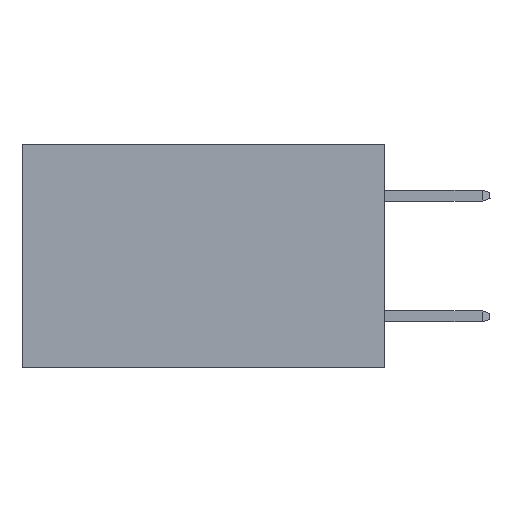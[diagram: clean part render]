
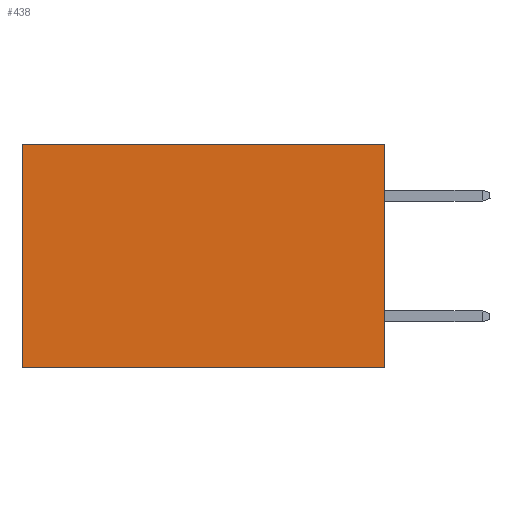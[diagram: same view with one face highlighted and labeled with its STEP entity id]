
A CAD part, left-side view. The second image highlights one B-rep face of the part: STEP entity #438.
In plain terms, the highlighted planar face has unit normal (-1, 0, 0).
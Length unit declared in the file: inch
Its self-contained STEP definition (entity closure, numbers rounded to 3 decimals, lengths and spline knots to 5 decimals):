
#314 = LINE ( 'NONE', #13650, #6365 ) ;
#370 = DIRECTION ( 'NONE',  ( 0., 1., 0. ) ) ;
#438 = ADVANCED_FACE ( 'NONE', ( #1884 ), #11918, .F. ) ;
#947 = CARTESIAN_POINT ( 'NONE',  ( 0.298, 0.6, 0. ) ) ;
#1336 = ORIENTED_EDGE ( 'NONE', *, *, #12572, .F. ) ;
#1884 = FACE_OUTER_BOUND ( 'NONE', #7012, .T. ) ;
#2105 = CARTESIAN_POINT ( 'NONE',  ( 0.298, 0.6, 0. ) ) ;
#2385 = VECTOR ( 'NONE', #9406, 39.37008 ) ;
#2459 = ORIENTED_EDGE ( 'NONE', *, *, #11567, .T. ) ;
#4093 = CARTESIAN_POINT ( 'NONE',  ( 0.298, 0., -0.37 ) ) ;
#4707 = VECTOR ( 'NONE', #14517, 39.37008 ) ;
#4843 = LINE ( 'NONE', #4093, #15502 ) ;
#4847 = DIRECTION ( 'NONE',  ( 0., 0., -1. ) ) ;
#5023 = CARTESIAN_POINT ( 'NONE',  ( 0.298, 0., -0.37 ) ) ;
#6365 = VECTOR ( 'NONE', #12545, 39.37008 ) ;
#6656 = VERTEX_POINT ( 'NONE', #5023 ) ;
#6680 = VERTEX_POINT ( 'NONE', #7475 ) ;
#6783 = LINE ( 'NONE', #9624, #4707 ) ;
#7012 = EDGE_LOOP ( 'NONE', ( #2459, #1336, #11537, #7087 ) ) ;
#7087 = ORIENTED_EDGE ( 'NONE', *, *, #10410, .T. ) ;
#7222 = CARTESIAN_POINT ( 'NONE',  ( 0.298, 0., 0. ) ) ;
#7475 = CARTESIAN_POINT ( 'NONE',  ( 0.298, 0.6, -0.37 ) ) ;
#9406 = DIRECTION ( 'NONE',  ( 0., 0., -1. ) ) ;
#9624 = CARTESIAN_POINT ( 'NONE',  ( 0.298, 0., 0. ) ) ;
#10410 = EDGE_CURVE ( 'NONE', #11607, #10759, #6783, .T. ) ;
#10686 = CARTESIAN_POINT ( 'NONE',  ( 0.298, 0., 0. ) ) ;
#10759 = VERTEX_POINT ( 'NONE', #2105 ) ;
#10783 = DIRECTION ( 'NONE',  ( 1., 0., 0. ) ) ;
#11267 = EDGE_CURVE ( 'NONE', #11607, #6656, #314, .T. ) ;
#11537 = ORIENTED_EDGE ( 'NONE', *, *, #11267, .F. ) ;
#11567 = EDGE_CURVE ( 'NONE', #10759, #6680, #13683, .T. ) ;
#11607 = VERTEX_POINT ( 'NONE', #7222 ) ;
#11918 = PLANE ( 'NONE',  #12795 ) ;
#12545 = DIRECTION ( 'NONE',  ( 0., 0., -1. ) ) ;
#12572 = EDGE_CURVE ( 'NONE', #6656, #6680, #4843, .T. ) ;
#12795 = AXIS2_PLACEMENT_3D ( 'NONE', #10686, #10783, #4847 ) ;
#13650 = CARTESIAN_POINT ( 'NONE',  ( 0.298, 0., 0. ) ) ;
#13683 = LINE ( 'NONE', #947, #2385 ) ;
#14517 = DIRECTION ( 'NONE',  ( 0., 1., 0. ) ) ;
#15502 = VECTOR ( 'NONE', #370, 39.37008 ) ;
